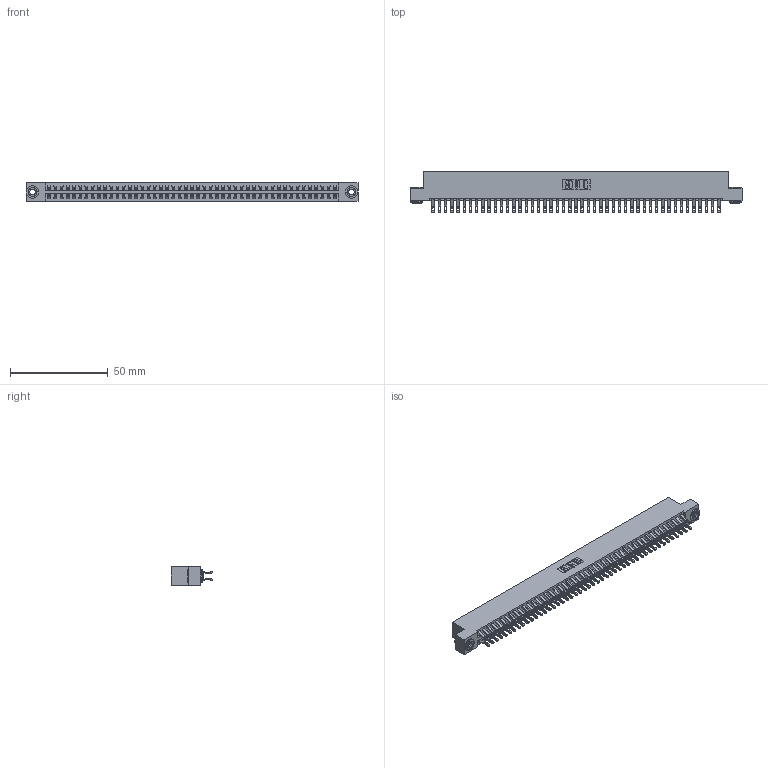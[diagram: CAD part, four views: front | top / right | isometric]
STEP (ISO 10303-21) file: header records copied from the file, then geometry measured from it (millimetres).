
FILE_DESCRIPTION (( 'STEP AP203' ), '1' );
FILE_NAME ('346-094-555-203.STEP', '2022-05-26T14:51:07', ( '' ), ( '' ), 'SwSTEP 2.0', 'SolidWorks 2020', '' );
FILE_SCHEMA (( 'CONFIG_CONTROL_DESIGN' ));
Length unit declared in the file: inch
Products named in the file (4): 345-250-002_345-250-002-102; 346-094-555-203; 345-292-001_555 Tail; 346 Part_Flush Mounting Lugs - 0.156 Dia-TH
Assembly tree (97 placements, depth 2):
  346-094-555-203
    346 Part_Flush Mounting Lugs - 0.156 Dia-TH
    345-292-001_555 Tail  x94
    345-250-002_345-250-002-102  x2
Bounding box: 169.8 x 21.46 x 9.4 mm (x, y, z)
Volume: 16870.3 mm3; surface area: 24488.6 mm2
Topology: 97 solids, 97 shells, 5626 faces, 17643 edges, 11758 vertices
Faces by surface type: plane 3202, cylinder 2416, cone 8
Entity records: 31392 total; most frequent: CARTESIAN_POINT 5183, ORIENTED_EDGE 5078, DIRECTION 4617, EDGE_CURVE 2539, LINE 2175, VECTOR 2175, VERTEX_POINT 1690, AXIS2_PLACEMENT_3D 1221
